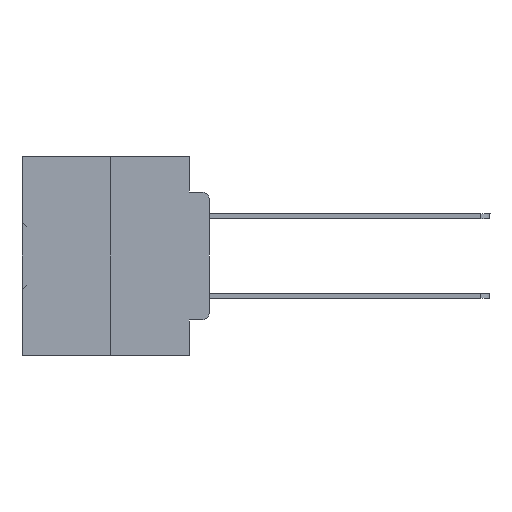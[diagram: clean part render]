
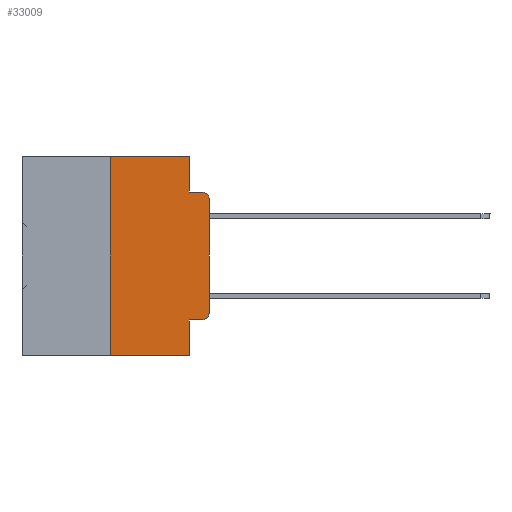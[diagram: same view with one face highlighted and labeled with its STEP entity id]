
A CAD part, left-side view. The second image highlights one B-rep face of the part: STEP entity #33009.
In plain terms, the highlighted planar face has unit normal (-1, 0, 0).
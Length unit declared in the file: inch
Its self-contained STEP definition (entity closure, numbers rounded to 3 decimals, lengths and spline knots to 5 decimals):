
#1452 = VECTOR ( 'NONE', #31818, 39.37008 ) ;
#1690 = VECTOR ( 'NONE', #4896, 39.37008 ) ;
#1978 = CARTESIAN_POINT ( 'NONE',  ( 0., 0.051, -0.4115 ) ) ;
#2958 = EDGE_CURVE ( 'NONE', #14687, #19679, #38185, .T. ) ;
#3990 = DIRECTION ( 'NONE',  ( 1., 0., 0. ) ) ;
#4896 = DIRECTION ( 'NONE',  ( 0., -1., 0. ) ) ;
#5239 = ORIENTED_EDGE ( 'NONE', *, *, #27185, .F. ) ;
#5365 = DIRECTION ( 'NONE',  ( -1., 0., 0. ) ) ;
#5434 = EDGE_CURVE ( 'NONE', #32453, #20093, #15074, .T. ) ;
#5665 = ORIENTED_EDGE ( 'NONE', *, *, #35473, .T. ) ;
#5687 = EDGE_CURVE ( 'NONE', #14687, #22735, #25810, .T. ) ;
#6399 = CARTESIAN_POINT ( 'NONE',  ( 0., 0.25, 0. ) ) ;
#6435 = CARTESIAN_POINT ( 'NONE',  ( 0., 0., 0. ) ) ;
#6584 = DIRECTION ( 'NONE',  ( 0., 0., -1. ) ) ;
#6613 = LINE ( 'NONE', #16732, #1452 ) ;
#7457 = AXIS2_PLACEMENT_3D ( 'NONE', #12092, #21497, #6584 ) ;
#7814 = VECTOR ( 'NONE', #24135, 39.37008 ) ;
#7851 = CARTESIAN_POINT ( 'NONE',  ( 0., 0.02, -0.3915 ) ) ;
#8640 = VERTEX_POINT ( 'NONE', #26152 ) ;
#8746 = LINE ( 'NONE', #36240, #7814 ) ;
#10383 = VERTEX_POINT ( 'NONE', #14511 ) ;
#10394 = ORIENTED_EDGE ( 'NONE', *, *, #18765, .F. ) ;
#10461 = CARTESIAN_POINT ( 'NONE',  ( 0., 0.25, -0.5 ) ) ;
#10464 = FACE_OUTER_BOUND ( 'NONE', #19550, .T. ) ;
#11091 = AXIS2_PLACEMENT_3D ( 'NONE', #7851, #5365, #16988 ) ;
#11756 = CIRCLE ( 'NONE', #7457, 0.02 ) ;
#11913 = CARTESIAN_POINT ( 'NONE',  ( 0., 0.051, -0.0885 ) ) ;
#12092 = CARTESIAN_POINT ( 'NONE',  ( 0., 0.02, -0.1085 ) ) ;
#12253 = EDGE_CURVE ( 'NONE', #18147, #32474, #38775, .T. ) ;
#12333 = DIRECTION ( 'NONE',  ( 0., 0., 1. ) ) ;
#12911 = CARTESIAN_POINT ( 'NONE',  ( 0., 0.051, -0.4115 ) ) ;
#13905 = DIRECTION ( 'NONE',  ( 0., 0., 1. ) ) ;
#14511 = CARTESIAN_POINT ( 'NONE',  ( 0., 0.051, -0.0885 ) ) ;
#14546 = DIRECTION ( 'NONE',  ( 0., -1., 0. ) ) ;
#14687 = VERTEX_POINT ( 'NONE', #10461 ) ;
#15074 = LINE ( 'NONE', #6435, #30556 ) ;
#16026 = CARTESIAN_POINT ( 'NONE',  ( 0., 0.473, 0. ) ) ;
#16732 = CARTESIAN_POINT ( 'NONE',  ( 0., 0.051, 0. ) ) ;
#16988 = DIRECTION ( 'NONE',  ( 0., 0., -1. ) ) ;
#17327 = CIRCLE ( 'NONE', #11091, 0.02 ) ;
#17350 = VECTOR ( 'NONE', #19746, 39.37008 ) ;
#17532 = ORIENTED_EDGE ( 'NONE', *, *, #5687, .T. ) ;
#17565 = VECTOR ( 'NONE', #32371, 39.37008 ) ;
#18057 = CARTESIAN_POINT ( 'NONE',  ( 0., 0.02, -0.0885 ) ) ;
#18147 = VERTEX_POINT ( 'NONE', #12911 ) ;
#18765 = EDGE_CURVE ( 'NONE', #10383, #20919, #27422, .T. ) ;
#19550 = EDGE_LOOP ( 'NONE', ( #33416, #5665, #10394, #30141, #5239, #30935, #17532, #38545, #38587, #20852 ) ) ;
#19679 = VERTEX_POINT ( 'NONE', #6399 ) ;
#19746 = DIRECTION ( 'NONE',  ( 0., -1., 0. ) ) ;
#20093 = VERTEX_POINT ( 'NONE', #20346 ) ;
#20328 = VECTOR ( 'NONE', #14546, 39.37008 ) ;
#20346 = CARTESIAN_POINT ( 'NONE',  ( 0., 0., -0.1085 ) ) ;
#20565 = EDGE_CURVE ( 'NONE', #8640, #10383, #6613, .T. ) ;
#20852 = ORIENTED_EDGE ( 'NONE', *, *, #28385, .T. ) ;
#20919 = VERTEX_POINT ( 'NONE', #18057 ) ;
#21497 = DIRECTION ( 'NONE',  ( -1., 0., 0. ) ) ;
#22735 = VERTEX_POINT ( 'NONE', #33298 ) ;
#24092 = VECTOR ( 'NONE', #13905, 39.37008 ) ;
#24135 = DIRECTION ( 'NONE',  ( 0., 0., -1. ) ) ;
#25788 = CARTESIAN_POINT ( 'NONE',  ( 0., 0., -0.3915 ) ) ;
#25810 = LINE ( 'NONE', #34481, #17350 ) ;
#25904 = EDGE_CURVE ( 'NONE', #18147, #22735, #8746, .T. ) ;
#26152 = CARTESIAN_POINT ( 'NONE',  ( 0., 0.051, 0. ) ) ;
#27185 = EDGE_CURVE ( 'NONE', #19679, #8640, #27916, .T. ) ;
#27422 = LINE ( 'NONE', #11913, #20328 ) ;
#27916 = LINE ( 'NONE', #38035, #17565 ) ;
#28385 = EDGE_CURVE ( 'NONE', #32474, #32453, #17327, .T. ) ;
#28905 = CARTESIAN_POINT ( 'NONE',  ( 0., 0.02, -0.4115 ) ) ;
#30141 = ORIENTED_EDGE ( 'NONE', *, *, #20565, .F. ) ;
#30556 = VECTOR ( 'NONE', #12333, 39.37008 ) ;
#30835 = PLANE ( 'NONE',  #36829 ) ;
#30935 = ORIENTED_EDGE ( 'NONE', *, *, #2958, .F. ) ;
#31087 = DIRECTION ( 'NONE',  ( 0., 0., -1. ) ) ;
#31588 = CARTESIAN_POINT ( 'NONE',  ( 0., 0.25, 0. ) ) ;
#31818 = DIRECTION ( 'NONE',  ( 0., 0., -1. ) ) ;
#32371 = DIRECTION ( 'NONE',  ( 0., -1., 0. ) ) ;
#32453 = VERTEX_POINT ( 'NONE', #25788 ) ;
#32474 = VERTEX_POINT ( 'NONE', #28905 ) ;
#33009 = ADVANCED_FACE ( 'NONE', ( #10464 ), #30835, .F. ) ;
#33298 = CARTESIAN_POINT ( 'NONE',  ( 0., 0.051, -0.5 ) ) ;
#33416 = ORIENTED_EDGE ( 'NONE', *, *, #5434, .T. ) ;
#34481 = CARTESIAN_POINT ( 'NONE',  ( 0., 0.473, -0.5 ) ) ;
#35473 = EDGE_CURVE ( 'NONE', #20093, #20919, #11756, .T. ) ;
#36240 = CARTESIAN_POINT ( 'NONE',  ( 0., 0.051, 0. ) ) ;
#36829 = AXIS2_PLACEMENT_3D ( 'NONE', #16026, #3990, #31087 ) ;
#38035 = CARTESIAN_POINT ( 'NONE',  ( 0., 0.473, 0. ) ) ;
#38185 = LINE ( 'NONE', #31588, #24092 ) ;
#38545 = ORIENTED_EDGE ( 'NONE', *, *, #25904, .F. ) ;
#38587 = ORIENTED_EDGE ( 'NONE', *, *, #12253, .T. ) ;
#38775 = LINE ( 'NONE', #1978, #1690 ) ;
